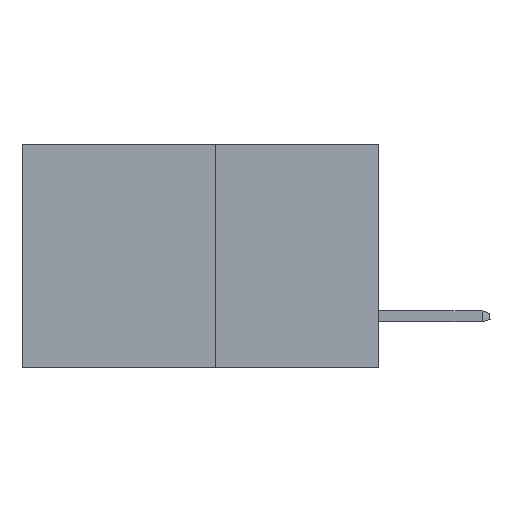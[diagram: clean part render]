
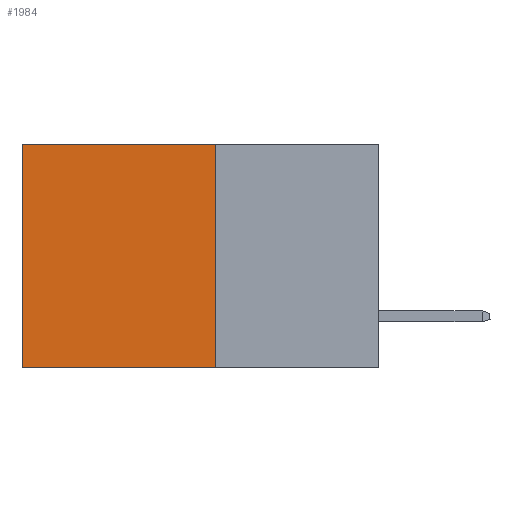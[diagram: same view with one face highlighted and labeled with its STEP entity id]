
A CAD part, left-side view. The second image highlights one B-rep face of the part: STEP entity #1984.
In plain terms, the highlighted planar face has unit normal (-1, 0, 0).
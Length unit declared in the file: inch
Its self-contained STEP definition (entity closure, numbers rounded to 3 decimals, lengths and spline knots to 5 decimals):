
#78 = DIRECTION ( 'NONE',  ( 0., 0., -1. ) ) ;
#183 = CARTESIAN_POINT ( 'NONE',  ( 0.277, 0.59, -0.37 ) ) ;
#592 = VECTOR ( 'NONE', #31502, 39.37008 ) ;
#955 = ORIENTED_EDGE ( 'NONE', *, *, #3412, .T. ) ;
#1984 = ADVANCED_FACE ( 'NONE', ( #31053 ), #7713, .F. ) ;
#3375 = CARTESIAN_POINT ( 'NONE',  ( 0.277, 0.27, -0.37 ) ) ;
#3412 = EDGE_CURVE ( 'NONE', #26147, #6287, #4430, .T. ) ;
#4211 = EDGE_CURVE ( 'NONE', #6287, #18119, #12552, .T. ) ;
#4430 = LINE ( 'NONE', #7002, #11049 ) ;
#5164 = ORIENTED_EDGE ( 'NONE', *, *, #30144, .F. ) ;
#5527 = CARTESIAN_POINT ( 'NONE',  ( 0.277, 0.59, 0. ) ) ;
#5897 = DIRECTION ( 'NONE',  ( 0., 1., 0. ) ) ;
#6287 = VERTEX_POINT ( 'NONE', #5527 ) ;
#7002 = CARTESIAN_POINT ( 'NONE',  ( 0.277, 0.27, 0. ) ) ;
#7113 = DIRECTION ( 'NONE',  ( 0., 1., 0. ) ) ;
#7713 = PLANE ( 'NONE',  #30288 ) ;
#10620 = CARTESIAN_POINT ( 'NONE',  ( 0.277, 0.27, 0. ) ) ;
#11049 = VECTOR ( 'NONE', #7113, 39.37008 ) ;
#12552 = LINE ( 'NONE', #183, #15478 ) ;
#15274 = CARTESIAN_POINT ( 'NONE',  ( 0.277, 0.27, -0.37 ) ) ;
#15478 = VECTOR ( 'NONE', #78, 39.37008 ) ;
#15738 = VECTOR ( 'NONE', #5897, 39.37008 ) ;
#16768 = CARTESIAN_POINT ( 'NONE',  ( 0.277, 0.27, -0.37 ) ) ;
#17112 = VERTEX_POINT ( 'NONE', #15274 ) ;
#18119 = VERTEX_POINT ( 'NONE', #18925 ) ;
#18925 = CARTESIAN_POINT ( 'NONE',  ( 0.277, 0.59, -0.37 ) ) ;
#18998 = EDGE_LOOP ( 'NONE', ( #19967, #5164, #26884, #955 ) ) ;
#19775 = DIRECTION ( 'NONE',  ( 0., 0., -1. ) ) ;
#19913 = DIRECTION ( 'NONE',  ( 1., 0., 0. ) ) ;
#19967 = ORIENTED_EDGE ( 'NONE', *, *, #4211, .T. ) ;
#20884 = EDGE_CURVE ( 'NONE', #26147, #17112, #26981, .T. ) ;
#26147 = VERTEX_POINT ( 'NONE', #10620 ) ;
#26884 = ORIENTED_EDGE ( 'NONE', *, *, #20884, .F. ) ;
#26981 = LINE ( 'NONE', #29065, #592 ) ;
#29065 = CARTESIAN_POINT ( 'NONE',  ( 0.277, 0.27, -0.37 ) ) ;
#29506 = LINE ( 'NONE', #3375, #15738 ) ;
#30144 = EDGE_CURVE ( 'NONE', #17112, #18119, #29506, .T. ) ;
#30288 = AXIS2_PLACEMENT_3D ( 'NONE', #16768, #19913, #19775 ) ;
#31053 = FACE_OUTER_BOUND ( 'NONE', #18998, .T. ) ;
#31502 = DIRECTION ( 'NONE',  ( 0., 0., -1. ) ) ;
